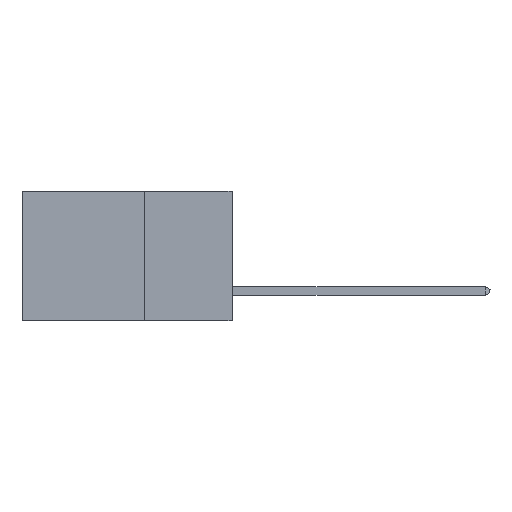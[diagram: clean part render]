
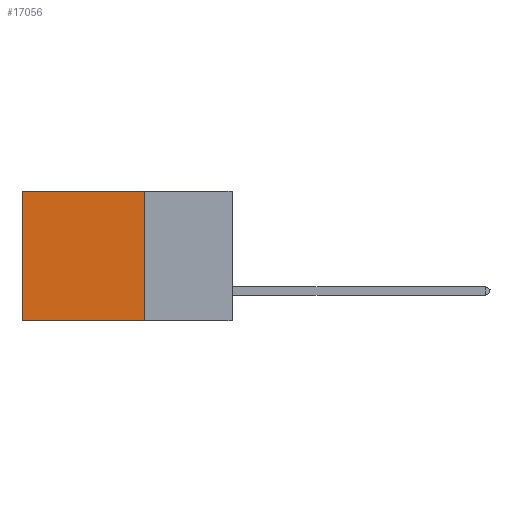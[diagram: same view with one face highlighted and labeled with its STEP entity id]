
A CAD part, left-side view. The second image highlights one B-rep face of the part: STEP entity #17056.
In plain terms, the highlighted planar face has unit normal (-1, 0, 0).
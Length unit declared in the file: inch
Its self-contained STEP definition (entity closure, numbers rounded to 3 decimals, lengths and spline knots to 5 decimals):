
#635 = AXIS2_PLACEMENT_3D ( 'NONE', #12472, #32212, #16688 ) ;
#3886 = VECTOR ( 'NONE', #22035, 39.37008 ) ;
#4406 = EDGE_CURVE ( 'NONE', #47985, #32759, #38066, .T. ) ;
#6174 = CARTESIAN_POINT ( 'NONE',  ( 0.2875, 0.6, 0. ) ) ;
#6314 = CARTESIAN_POINT ( 'NONE',  ( 0.2875, 0.6, 0. ) ) ;
#8436 = FACE_OUTER_BOUND ( 'NONE', #35388, .T. ) ;
#8630 = CARTESIAN_POINT ( 'NONE',  ( 0.2875, 0.25, -0.37 ) ) ;
#11017 = CARTESIAN_POINT ( 'NONE',  ( 0.2875, 0.25, 0. ) ) ;
#11090 = ORIENTED_EDGE ( 'NONE', *, *, #4406, .F. ) ;
#12472 = CARTESIAN_POINT ( 'NONE',  ( 0.2875, 0.25, 0. ) ) ;
#16688 = DIRECTION ( 'NONE',  ( 0., 0., -1. ) ) ;
#17056 = ADVANCED_FACE ( 'NONE', ( #8436 ), #20544, .F. ) ;
#17256 = VERTEX_POINT ( 'NONE', #6174 ) ;
#17864 = EDGE_CURVE ( 'NONE', #17256, #32759, #28848, .T. ) ;
#18096 = VECTOR ( 'NONE', #40729, 39.37008 ) ;
#19972 = VECTOR ( 'NONE', #36631, 39.37008 ) ;
#20544 = PLANE ( 'NONE',  #635 ) ;
#21067 = ORIENTED_EDGE ( 'NONE', *, *, #17864, .T. ) ;
#22035 = DIRECTION ( 'NONE',  ( 0., 1., 0. ) ) ;
#22598 = ORIENTED_EDGE ( 'NONE', *, *, #27828, .T. ) ;
#25284 = CARTESIAN_POINT ( 'NONE',  ( 0.2875, 0.6, -0.37 ) ) ;
#27828 = EDGE_CURVE ( 'NONE', #42699, #17256, #49265, .T. ) ;
#28848 = LINE ( 'NONE', #6314, #18096 ) ;
#32212 = DIRECTION ( 'NONE',  ( 1., 0., 0. ) ) ;
#32759 = VERTEX_POINT ( 'NONE', #25284 ) ;
#34860 = LINE ( 'NONE', #37115, #41473 ) ;
#35388 = EDGE_LOOP ( 'NONE', ( #21067, #11090, #40088, #22598 ) ) ;
#36631 = DIRECTION ( 'NONE',  ( 0., 1., 0. ) ) ;
#37115 = CARTESIAN_POINT ( 'NONE',  ( 0.2875, 0.25, 0. ) ) ;
#38066 = LINE ( 'NONE', #8630, #19972 ) ;
#40088 = ORIENTED_EDGE ( 'NONE', *, *, #44371, .F. ) ;
#40729 = DIRECTION ( 'NONE',  ( 0., 0., -1. ) ) ;
#41327 = CARTESIAN_POINT ( 'NONE',  ( 0.2875, 0.25, -0.37 ) ) ;
#41473 = VECTOR ( 'NONE', #44944, 39.37008 ) ;
#42699 = VERTEX_POINT ( 'NONE', #45825 ) ;
#44371 = EDGE_CURVE ( 'NONE', #42699, #47985, #34860, .T. ) ;
#44944 = DIRECTION ( 'NONE',  ( 0., 0., -1. ) ) ;
#45825 = CARTESIAN_POINT ( 'NONE',  ( 0.2875, 0.25, 0. ) ) ;
#47985 = VERTEX_POINT ( 'NONE', #41327 ) ;
#49265 = LINE ( 'NONE', #11017, #3886 ) ;
